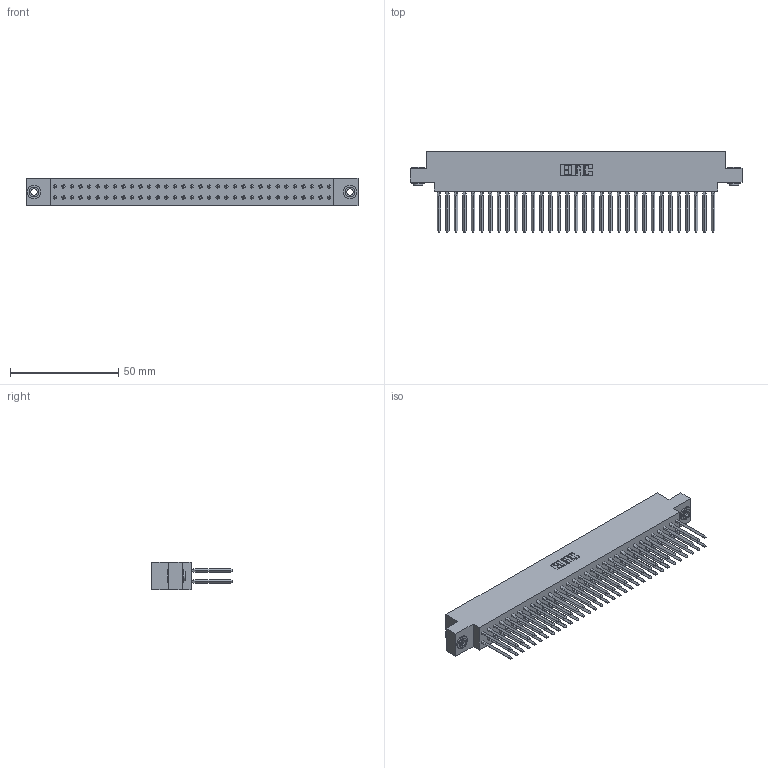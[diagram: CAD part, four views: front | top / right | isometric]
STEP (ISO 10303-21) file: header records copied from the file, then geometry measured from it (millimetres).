
FILE_DESCRIPTION (( 'STEP AP203' ), '1' );
FILE_NAME ('317-066-542-803.STEP', '2020-02-28T06:17:30', ( '' ), ( '' ), 'SwSTEP 2.0', 'SolidWorks 2016', '' );
FILE_SCHEMA (( 'CONFIG_CONTROL_DESIGN' ));
Length unit declared in the file: inch
Products named in the file (4): 317 Part_.156 Dia - TH; 317-290-003_542; 317-066-542-803; 345-250-002_345-250-002-102
Assembly tree (69 placements, depth 2):
  317-066-542-803
    317 Part_.156 Dia - TH
    317-290-003_542  x66
    345-250-002_345-250-002-102  x2
Bounding box: 153.47 x 37.34 x 12.7 mm (x, y, z)
Volume: 24864.6 mm3; surface area: 34504 mm2
Topology: 69 solids, 69 shells, 3902 faces, 10911 edges, 6962 vertices
Faces by surface type: plane 3104, cylinder 526, bspline 264, cone 8
Entity records: 48624 total; most frequent: CARTESIAN_POINT 8700, ORIENTED_EDGE 8356, DIRECTION 7084, EDGE_CURVE 4178, VECTOR 3984, LINE 3984, VERTEX_POINT 2778, AXIS2_PLACEMENT_3D 1550
